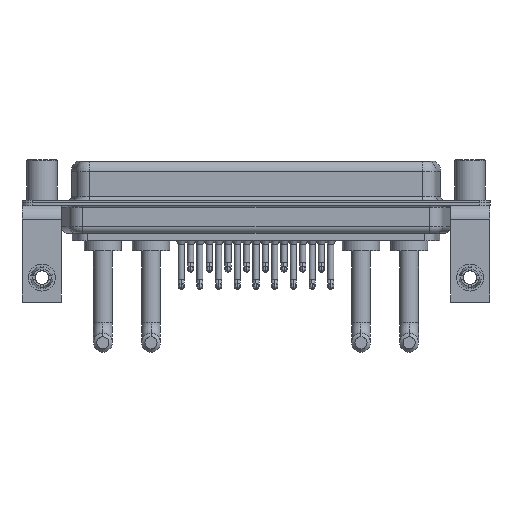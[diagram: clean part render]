
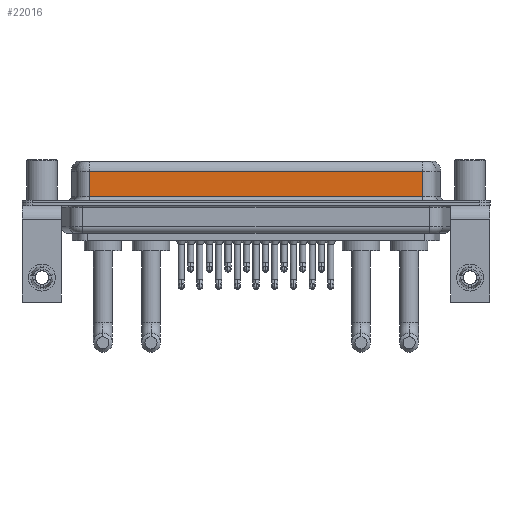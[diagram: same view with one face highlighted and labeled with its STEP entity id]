
A CAD part, front view. The second image highlights one B-rep face of the part: STEP entity #22016.
In plain terms, the highlighted planar face has unit normal (0, -1, 0).
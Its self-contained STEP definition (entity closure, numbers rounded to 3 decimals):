
#204 = EDGE_CURVE ( 'NONE', #17314, #16106, #11283, .T. ) ;
#630 = ORIENTED_EDGE ( 'NONE', *, *, #23197, .T. ) ;
#783 = VERTEX_POINT ( 'NONE', #25804 ) ;
#1352 = CARTESIAN_POINT ( 'NONE',  ( 7.038, -3.95, 6.4 ) ) ;
#1487 = VERTEX_POINT ( 'NONE', #4375 ) ;
#1870 = EDGE_CURVE ( 'NONE', #16106, #783, #11117, .T. ) ;
#2441 = CARTESIAN_POINT ( 'NONE',  ( 56.462, -3.95, 6.4 ) ) ;
#4074 = AXIS2_PLACEMENT_3D ( 'NONE', #24482, #8958, #13055 ) ;
#4375 = CARTESIAN_POINT ( 'NONE',  ( 56.462, -3.95, 4.65 ) ) ;
#5834 = DIRECTION ( 'NONE',  ( 0., 0., -1. ) ) ;
#6799 = LINE ( 'NONE', #2441, #21926 ) ;
#7551 = ORIENTED_EDGE ( 'NONE', *, *, #14754, .F. ) ;
#8199 = FACE_OUTER_BOUND ( 'NONE', #15160, .T. ) ;
#8958 = DIRECTION ( 'NONE',  ( 0., 1., 0. ) ) ;
#10207 = CARTESIAN_POINT ( 'NONE',  ( 56.462, -3.95, 4.65 ) ) ;
#11117 = LINE ( 'NONE', #17757, #20967 ) ;
#11283 = LINE ( 'NONE', #1352, #17195 ) ;
#11368 = CARTESIAN_POINT ( 'NONE',  ( 7.038, -3.95, 4.65 ) ) ;
#11386 = DIRECTION ( 'NONE',  ( 1., 0., 0. ) ) ;
#12754 = DIRECTION ( 'NONE',  ( 0., 0., -1. ) ) ;
#13055 = DIRECTION ( 'NONE',  ( 0., 0., 1. ) ) ;
#14754 = EDGE_CURVE ( 'NONE', #1487, #783, #6799, .T. ) ;
#15160 = EDGE_LOOP ( 'NONE', ( #7551, #630, #17614, #22668 ) ) ;
#16106 = VERTEX_POINT ( 'NONE', #22822 ) ;
#16536 = PLANE ( 'NONE',  #4074 ) ;
#17195 = VECTOR ( 'NONE', #5834, 1000. ) ;
#17314 = VERTEX_POINT ( 'NONE', #11368 ) ;
#17614 = ORIENTED_EDGE ( 'NONE', *, *, #204, .T. ) ;
#17757 = CARTESIAN_POINT ( 'NONE',  ( 56.462, -3.95, 0.9 ) ) ;
#20967 = VECTOR ( 'NONE', #11386, 1000. ) ;
#21049 = VECTOR ( 'NONE', #22096, 1000. ) ;
#21926 = VECTOR ( 'NONE', #12754, 1000. ) ;
#22016 = ADVANCED_FACE ( 'NONE', ( #8199 ), #16536, .F. ) ;
#22096 = DIRECTION ( 'NONE',  ( -1., 0., 0. ) ) ;
#22668 = ORIENTED_EDGE ( 'NONE', *, *, #1870, .T. ) ;
#22822 = CARTESIAN_POINT ( 'NONE',  ( 7.038, -3.95, 0.9 ) ) ;
#23197 = EDGE_CURVE ( 'NONE', #1487, #17314, #24093, .T. ) ;
#24093 = LINE ( 'NONE', #10207, #21049 ) ;
#24482 = CARTESIAN_POINT ( 'NONE',  ( 56.462, -3.95, 6.4 ) ) ;
#25804 = CARTESIAN_POINT ( 'NONE',  ( 56.462, -3.95, 0.9 ) ) ;
